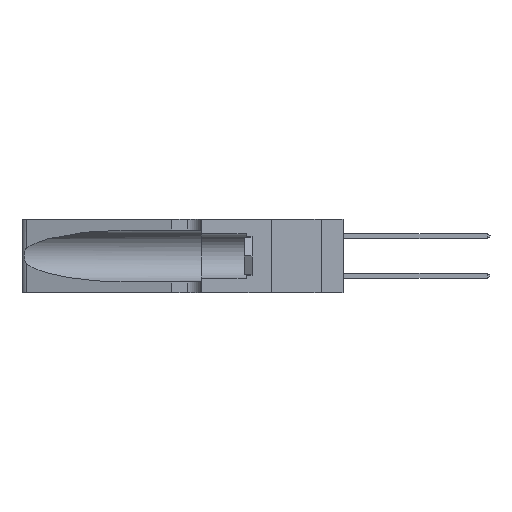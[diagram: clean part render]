
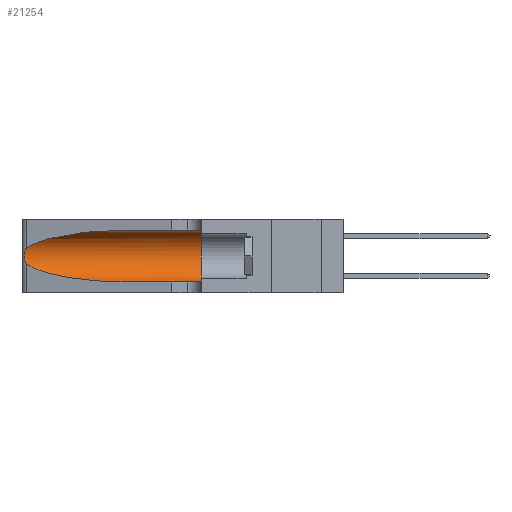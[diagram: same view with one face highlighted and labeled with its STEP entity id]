
A CAD part, left-side view. The second image highlights one B-rep face of the part: STEP entity #21254.
In plain terms, the highlighted cylindrical face has radius 3.308 mm (diameter 6.617 mm), a partial arc.
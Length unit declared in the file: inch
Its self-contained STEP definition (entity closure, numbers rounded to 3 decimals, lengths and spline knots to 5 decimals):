
#409 = ORIENTED_EDGE ( 'NONE', *, *, #18753, .F. ) ;
#1105 = CYLINDRICAL_SURFACE ( 'NONE', #31820, 0.13025 ) ;
#1772 = CARTESIAN_POINT ( 'NONE',  ( 0.18966, 0.96281, 0.05475 ) ) ;
#1945 = VECTOR ( 'NONE', #46255, 39.37008 ) ;
#2270 = FACE_OUTER_BOUND ( 'NONE', #37726, .T. ) ;
#2404 = CARTESIAN_POINT ( 'NONE',  ( 0.25487, 1.22718, 0.22369 ) ) ;
#2560 = CARTESIAN_POINT ( 'NONE',  ( 0.25639, 1.23186, 0.15144 ) ) ;
#3130 = EDGE_CURVE ( 'NONE', #29966, #21748, #5170, .T. ) ;
#3869 = ORIENTED_EDGE ( 'NONE', *, *, #6396, .F. ) ;
#4448 = CARTESIAN_POINT ( 'NONE',  ( 0.1305, 1.61858, 0.05475 ) ) ;
#5170 =( BOUNDED_CURVE ( )  B_SPLINE_CURVE ( 3, ( #27298, #23630, #1772, #5449 ),
 .UNSPECIFIED., .F., .T. ) 
 B_SPLINE_CURVE_WITH_KNOTS ( ( 4, 4 ),
 ( 3.44316, 4.71239 ),
 .UNSPECIFIED. ) 
 CURVE ( )  GEOMETRIC_REPRESENTATION_ITEM ( )  RATIONAL_B_SPLINE_CURVE ( ( 1., 0.87, 0.87, 1. ) ) 
 REPRESENTATION_ITEM ( '' )  );
#5449 = CARTESIAN_POINT ( 'NONE',  ( 0.1305, 0.72297, 0.05475 ) ) ;
#6248 = CARTESIAN_POINT ( 'NONE',  ( 0.25487, 1.22718, 0.14631 ) ) ;
#6396 = EDGE_CURVE ( 'NONE', #43023, #20595, #20228, .T. ) ;
#6586 = CARTESIAN_POINT ( 'NONE',  ( 0.18966, 0.96281, 0.31525 ) ) ;
#7600 = EDGE_CURVE ( 'NONE', #22402, #29966, #29753, .T. ) ;
#8138 = DIRECTION ( 'NONE',  ( 0., -1., 0. ) ) ;
#9245 = VERTEX_POINT ( 'NONE', #23559 ) ;
#9314 =( BOUNDED_CURVE ( )  B_SPLINE_CURVE ( 3, ( #28274, #6586, #10291, #35704 ),
 .UNSPECIFIED., .F., .T. ) 
 B_SPLINE_CURVE_WITH_KNOTS ( ( 4, 4 ),
 ( 1.5708, 2.84003 ),
 .UNSPECIFIED. ) 
 CURVE ( )  GEOMETRIC_REPRESENTATION_ITEM ( )  RATIONAL_B_SPLINE_CURVE ( ( 1., 0.87, 0.87, 1. ) ) 
 REPRESENTATION_ITEM ( '' )  );
#9780 = CARTESIAN_POINT ( 'NONE',  ( 0.25639, 1.23184, 0.21858 ) ) ;
#10291 = CARTESIAN_POINT ( 'NONE',  ( 0.2373, 1.15595, 0.28018 ) ) ;
#10761 = DIRECTION ( 'NONE',  ( 0., 0., -1. ) ) ;
#10945 = EDGE_CURVE ( 'NONE', #21748, #9245, #35510, .T. ) ;
#12945 = ORIENTED_EDGE ( 'NONE', *, *, #10945, .T. ) ;
#13405 = CARTESIAN_POINT ( 'NONE',  ( 0.25854, 1.2359, 0.20912 ) ) ;
#14409 = CARTESIAN_POINT ( 'NONE',  ( 0.1305, 1.61858, 0.185 ) ) ;
#15083 = DIRECTION ( 'NONE',  ( 0., 1., 0. ) ) ;
#16176 = VECTOR ( 'NONE', #8138, 39.37008 ) ;
#16200 = AXIS2_PLACEMENT_3D ( 'NONE', #36831, #15083, #40438 ) ;
#17114 = CARTESIAN_POINT ( 'NONE',  ( 0.26075, 1.23896, 0.19203 ) ) ;
#18668 = ORIENTED_EDGE ( 'NONE', *, *, #19232, .T. ) ;
#18753 = EDGE_CURVE ( 'NONE', #20595, #9245, #45801, .T. ) ;
#19221 = CARTESIAN_POINT ( 'NONE',  ( 0.1305, 0.72297, 0.05475 ) ) ;
#19232 = EDGE_CURVE ( 'NONE', #43023, #22402, #9314, .T. ) ;
#20228 = LINE ( 'NONE', #21022, #1945 ) ;
#20595 = VERTEX_POINT ( 'NONE', #35752 ) ;
#20612 = CARTESIAN_POINT ( 'NONE',  ( 0.25555, 1.22994, 0.2215 ) ) ;
#20761 = CARTESIAN_POINT ( 'NONE',  ( 0.26017, 1.23833, 0.17102 ) ) ;
#21022 = CARTESIAN_POINT ( 'NONE',  ( 0.1305, 1.61858, 0.31525 ) ) ;
#21254 = ADVANCED_FACE ( 'NONE', ( #2270 ), #1105, .F. ) ;
#21589 = DIRECTION ( 'NONE',  ( 0., -1., 0. ) ) ;
#21748 = VERTEX_POINT ( 'NONE', #19221 ) ;
#22402 = VERTEX_POINT ( 'NONE', #26485 ) ;
#23559 = CARTESIAN_POINT ( 'NONE',  ( 0.1305, 0.35, 0.05475 ) ) ;
#23630 = CARTESIAN_POINT ( 'NONE',  ( 0.2373, 1.15595, 0.08982 ) ) ;
#24414 = CARTESIAN_POINT ( 'NONE',  ( 0.25789, 1.23486, 0.15765 ) ) ;
#26485 = CARTESIAN_POINT ( 'NONE',  ( 0.25487, 1.22718, 0.22369 ) ) ;
#27298 = CARTESIAN_POINT ( 'NONE',  ( 0.25487, 1.22718, 0.14631 ) ) ;
#28087 = CARTESIAN_POINT ( 'NONE',  ( 0.25555, 1.22993, 0.14849 ) ) ;
#28274 = CARTESIAN_POINT ( 'NONE',  ( 0.1305, 0.72297, 0.31525 ) ) ;
#29753 = B_SPLINE_CURVE_WITH_KNOTS ( 'NONE', 3,
 ( #2404, #20612, #9780, #35211, #13405, #38821, #17114, #42389, #20761, #46008, #24414, #2560, #28087, #6248 ),
 .UNSPECIFIED., .F., .F.,
 ( 4, 2, 2, 2, 2, 2, 4 ),
 ( 0., 0.00027, 0.00053, 0.00107, 0.0016, 0.00187, 0.00214 ),
 .UNSPECIFIED. ) ;
#29966 = VERTEX_POINT ( 'NONE', #30016 ) ;
#30016 = CARTESIAN_POINT ( 'NONE',  ( 0.25487, 1.22718, 0.14631 ) ) ;
#31820 = AXIS2_PLACEMENT_3D ( 'NONE', #14409, #21589, #10761 ) ;
#34001 = ORIENTED_EDGE ( 'NONE', *, *, #7600, .T. ) ;
#35211 = CARTESIAN_POINT ( 'NONE',  ( 0.25787, 1.23484, 0.2124 ) ) ;
#35510 = LINE ( 'NONE', #4448, #16176 ) ;
#35704 = CARTESIAN_POINT ( 'NONE',  ( 0.25487, 1.22718, 0.22369 ) ) ;
#35752 = CARTESIAN_POINT ( 'NONE',  ( 0.1305, 0.35, 0.31525 ) ) ;
#36831 = CARTESIAN_POINT ( 'NONE',  ( 0.1305, 0.35, 0.185 ) ) ;
#36968 = CARTESIAN_POINT ( 'NONE',  ( 0.1305, 0.72297, 0.31525 ) ) ;
#37726 = EDGE_LOOP ( 'NONE', ( #18668, #34001, #46935, #12945, #409, #3869 ) ) ;
#38821 = CARTESIAN_POINT ( 'NONE',  ( 0.26018, 1.23835, 0.19895 ) ) ;
#40438 = DIRECTION ( 'NONE',  ( 0., 0., 1. ) ) ;
#42389 = CARTESIAN_POINT ( 'NONE',  ( 0.26075, 1.23896, 0.178 ) ) ;
#43023 = VERTEX_POINT ( 'NONE', #36968 ) ;
#45801 = CIRCLE ( 'NONE', #16200, 0.13025 ) ;
#46008 = CARTESIAN_POINT ( 'NONE',  ( 0.25856, 1.23593, 0.16098 ) ) ;
#46255 = DIRECTION ( 'NONE',  ( 0., -1., 0. ) ) ;
#46935 = ORIENTED_EDGE ( 'NONE', *, *, #3130, .T. ) ;
